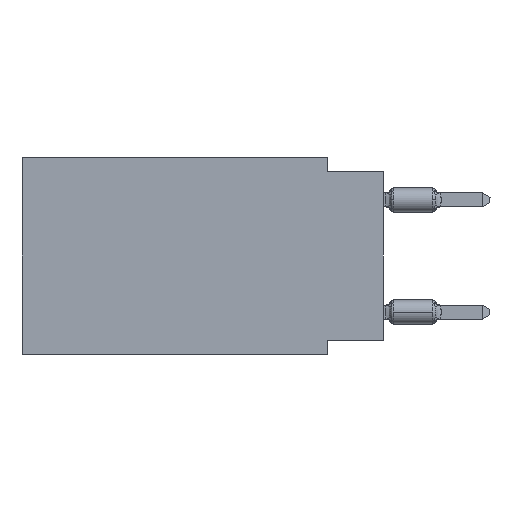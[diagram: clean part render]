
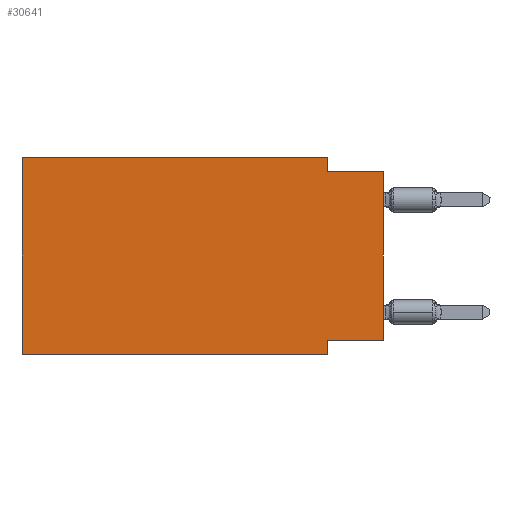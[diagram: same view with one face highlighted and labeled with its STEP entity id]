
A CAD part, left-side view. The second image highlights one B-rep face of the part: STEP entity #30641.
In plain terms, the highlighted planar face has unit normal (-1, 0, 0).
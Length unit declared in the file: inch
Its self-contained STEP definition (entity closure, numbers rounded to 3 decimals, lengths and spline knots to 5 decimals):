
#520 = VERTEX_POINT ( 'NONE', #54705 ) ;
#1867 = LINE ( 'NONE', #24109, #37228 ) ;
#1946 = DIRECTION ( 'NONE',  ( 0., 0., -1. ) ) ;
#1996 = EDGE_CURVE ( 'NONE', #42628, #23884, #1867, .T. ) ;
#3499 = ORIENTED_EDGE ( 'NONE', *, *, #11994, .F. ) ;
#7259 = DIRECTION ( 'NONE',  ( 0., -1., 0. ) ) ;
#7765 = LINE ( 'NONE', #40980, #54268 ) ;
#10244 = ORIENTED_EDGE ( 'NONE', *, *, #20495, .F. ) ;
#10614 = ORIENTED_EDGE ( 'NONE', *, *, #71162, .T. ) ;
#11264 = EDGE_CURVE ( 'NONE', #70144, #58231, #32539, .T. ) ;
#11994 = EDGE_CURVE ( 'NONE', #520, #70144, #36058, .T. ) ;
#12595 = VERTEX_POINT ( 'NONE', #38156 ) ;
#17503 = VECTOR ( 'NONE', #44381, 39.37008 ) ;
#17912 = CARTESIAN_POINT ( 'NONE',  ( 0., 0., -0.025 ) ) ;
#18875 = CARTESIAN_POINT ( 'NONE',  ( 0., 0.1, -0.025 ) ) ;
#19482 = DIRECTION ( 'NONE',  ( 0., 1., 0. ) ) ;
#20495 = EDGE_CURVE ( 'NONE', #45879, #12595, #7765, .T. ) ;
#21609 = CARTESIAN_POINT ( 'NONE',  ( 0., 0.1, 0. ) ) ;
#22277 = ORIENTED_EDGE ( 'NONE', *, *, #22535, .F. ) ;
#22535 = EDGE_CURVE ( 'NONE', #58231, #23884, #49230, .T. ) ;
#23218 = VERTEX_POINT ( 'NONE', #43925 ) ;
#23884 = VERTEX_POINT ( 'NONE', #17912 ) ;
#24071 = EDGE_CURVE ( 'NONE', #23218, #520, #33794, .T. ) ;
#24109 = CARTESIAN_POINT ( 'NONE',  ( 0., 0., 0. ) ) ;
#24472 = VECTOR ( 'NONE', #71075, 39.37008 ) ;
#25820 = DIRECTION ( 'NONE',  ( 1., 0., 0. ) ) ;
#27185 = DIRECTION ( 'NONE',  ( 0., -1., 0. ) ) ;
#27265 = ORIENTED_EDGE ( 'NONE', *, *, #28776, .F. ) ;
#27660 = ORIENTED_EDGE ( 'NONE', *, *, #24071, .F. ) ;
#28776 = EDGE_CURVE ( 'NONE', #42628, #45879, #70150, .T. ) ;
#30641 = ADVANCED_FACE ( 'NONE', ( #69539 ), #31272, .F. ) ;
#30810 = AXIS2_PLACEMENT_3D ( 'NONE', #64453, #25820, #64080 ) ;
#31272 = PLANE ( 'NONE',  #30810 ) ;
#32539 = LINE ( 'NONE', #21609, #51481 ) ;
#33794 = LINE ( 'NONE', #49835, #17503 ) ;
#36058 = LINE ( 'NONE', #51408, #66501 ) ;
#37228 = VECTOR ( 'NONE', #46348, 39.37008 ) ;
#38156 = CARTESIAN_POINT ( 'NONE',  ( 0., 0.1, -0.35 ) ) ;
#40980 = CARTESIAN_POINT ( 'NONE',  ( 0., 0.1, -0.35 ) ) ;
#42486 = CARTESIAN_POINT ( 'NONE',  ( 0., 0., -0.325 ) ) ;
#42628 = VERTEX_POINT ( 'NONE', #66189 ) ;
#43925 = CARTESIAN_POINT ( 'NONE',  ( 0., 0.645, -0.35 ) ) ;
#44318 = LINE ( 'NONE', #55253, #55881 ) ;
#44381 = DIRECTION ( 'NONE',  ( 0., 0., 1. ) ) ;
#45879 = VERTEX_POINT ( 'NONE', #61528 ) ;
#46348 = DIRECTION ( 'NONE',  ( 0., 0., 1. ) ) ;
#47519 = ORIENTED_EDGE ( 'NONE', *, *, #1996, .T. ) ;
#49230 = LINE ( 'NONE', #59811, #24472 ) ;
#49332 = DIRECTION ( 'NONE',  ( 0., 0., -1. ) ) ;
#49835 = CARTESIAN_POINT ( 'NONE',  ( 0., 0.645, 0. ) ) ;
#50512 = EDGE_LOOP ( 'NONE', ( #47519, #22277, #53270, #3499, #27660, #10614, #10244, #27265 ) ) ;
#51408 = CARTESIAN_POINT ( 'NONE',  ( 0., 0.645, 0. ) ) ;
#51481 = VECTOR ( 'NONE', #49332, 39.37008 ) ;
#53270 = ORIENTED_EDGE ( 'NONE', *, *, #11264, .F. ) ;
#53706 = CARTESIAN_POINT ( 'NONE',  ( 0., 0.1, 0. ) ) ;
#54268 = VECTOR ( 'NONE', #1946, 39.37008 ) ;
#54705 = CARTESIAN_POINT ( 'NONE',  ( 0., 0.645, 0. ) ) ;
#55253 = CARTESIAN_POINT ( 'NONE',  ( 0., 0.645, -0.35 ) ) ;
#55881 = VECTOR ( 'NONE', #27185, 39.37008 ) ;
#58231 = VERTEX_POINT ( 'NONE', #18875 ) ;
#59811 = CARTESIAN_POINT ( 'NONE',  ( 0., 0., -0.025 ) ) ;
#61528 = CARTESIAN_POINT ( 'NONE',  ( 0., 0.1, -0.325 ) ) ;
#64026 = VECTOR ( 'NONE', #19482, 39.37008 ) ;
#64080 = DIRECTION ( 'NONE',  ( 0., 0., -1. ) ) ;
#64453 = CARTESIAN_POINT ( 'NONE',  ( 0., 0.645, 0. ) ) ;
#66189 = CARTESIAN_POINT ( 'NONE',  ( 0., 0., -0.325 ) ) ;
#66501 = VECTOR ( 'NONE', #7259, 39.37008 ) ;
#69539 = FACE_OUTER_BOUND ( 'NONE', #50512, .T. ) ;
#70144 = VERTEX_POINT ( 'NONE', #53706 ) ;
#70150 = LINE ( 'NONE', #42486, #64026 ) ;
#71075 = DIRECTION ( 'NONE',  ( 0., -1., 0. ) ) ;
#71162 = EDGE_CURVE ( 'NONE', #23218, #12595, #44318, .T. ) ;
